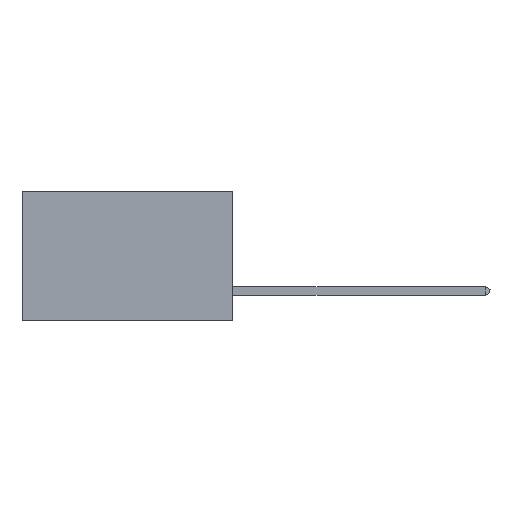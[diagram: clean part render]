
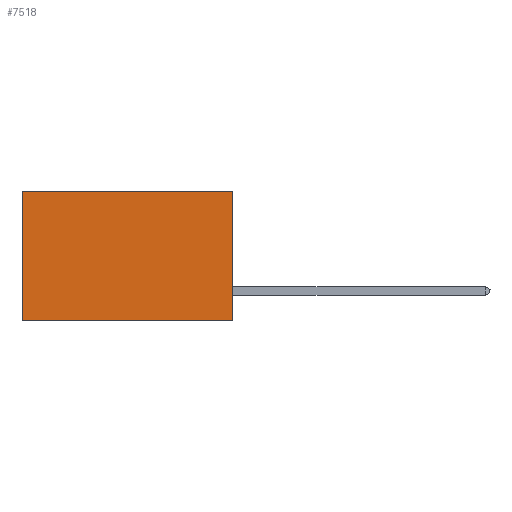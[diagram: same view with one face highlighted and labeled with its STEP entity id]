
A CAD part, left-side view. The second image highlights one B-rep face of the part: STEP entity #7518.
In plain terms, the highlighted planar face has unit normal (-1, 0, 0).
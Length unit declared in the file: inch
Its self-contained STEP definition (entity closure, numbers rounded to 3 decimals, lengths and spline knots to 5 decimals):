
#3349 = ORIENTED_EDGE ( 'NONE', *, *, #7915, .F. ) ;
#4034 = DIRECTION ( 'NONE',  ( 0., 0., -1. ) ) ;
#4268 = AXIS2_PLACEMENT_3D ( 'NONE', #34988, #4301, #4034 ) ;
#4301 = DIRECTION ( 'NONE',  ( 1., 0., 0. ) ) ;
#5522 = DIRECTION ( 'NONE',  ( 0., 0., -1. ) ) ;
#7518 = ADVANCED_FACE ( 'NONE', ( #11255 ), #28523, .F. ) ;
#7888 = EDGE_CURVE ( 'NONE', #33617, #38670, #35957, .T. ) ;
#7915 = EDGE_CURVE ( 'NONE', #10611, #29947, #29417, .T. ) ;
#8028 = CARTESIAN_POINT ( 'NONE',  ( 0.2875, 0.6, -0.37 ) ) ;
#10611 = VERTEX_POINT ( 'NONE', #32504 ) ;
#11255 = FACE_OUTER_BOUND ( 'NONE', #40214, .T. ) ;
#13104 = CARTESIAN_POINT ( 'NONE',  ( 0.2875, 0., 0. ) ) ;
#13499 = CARTESIAN_POINT ( 'NONE',  ( 0.2875, 0., 0. ) ) ;
#14759 = CARTESIAN_POINT ( 'NONE',  ( 0.2875, 0., -0.37 ) ) ;
#17414 = ORIENTED_EDGE ( 'NONE', *, *, #7888, .T. ) ;
#17990 = CARTESIAN_POINT ( 'NONE',  ( 0.2875, 0., 0. ) ) ;
#21105 = VECTOR ( 'NONE', #28777, 39.37008 ) ;
#25621 = LINE ( 'NONE', #37495, #21105 ) ;
#25885 = DIRECTION ( 'NONE',  ( 0., 1., 0. ) ) ;
#28523 = PLANE ( 'NONE',  #4268 ) ;
#28777 = DIRECTION ( 'NONE',  ( 0., 0., -1. ) ) ;
#29025 = ORIENTED_EDGE ( 'NONE', *, *, #38573, .T. ) ;
#29417 = LINE ( 'NONE', #14759, #40454 ) ;
#29947 = VERTEX_POINT ( 'NONE', #8028 ) ;
#32126 = EDGE_CURVE ( 'NONE', #33617, #10611, #40274, .T. ) ;
#32504 = CARTESIAN_POINT ( 'NONE',  ( 0.2875, 0., -0.37 ) ) ;
#33226 = DIRECTION ( 'NONE',  ( 0., 1., 0. ) ) ;
#33617 = VERTEX_POINT ( 'NONE', #13104 ) ;
#34988 = CARTESIAN_POINT ( 'NONE',  ( 0.2875, 0., 0. ) ) ;
#35287 = VECTOR ( 'NONE', #5522, 39.37008 ) ;
#35957 = LINE ( 'NONE', #13499, #40982 ) ;
#37495 = CARTESIAN_POINT ( 'NONE',  ( 0.2875, 0.6, 0. ) ) ;
#38467 = CARTESIAN_POINT ( 'NONE',  ( 0.2875, 0.6, 0. ) ) ;
#38573 = EDGE_CURVE ( 'NONE', #38670, #29947, #25621, .T. ) ;
#38670 = VERTEX_POINT ( 'NONE', #38467 ) ;
#40214 = EDGE_LOOP ( 'NONE', ( #29025, #3349, #40473, #17414 ) ) ;
#40274 = LINE ( 'NONE', #17990, #35287 ) ;
#40454 = VECTOR ( 'NONE', #33226, 39.37008 ) ;
#40473 = ORIENTED_EDGE ( 'NONE', *, *, #32126, .F. ) ;
#40982 = VECTOR ( 'NONE', #25885, 39.37008 ) ;
